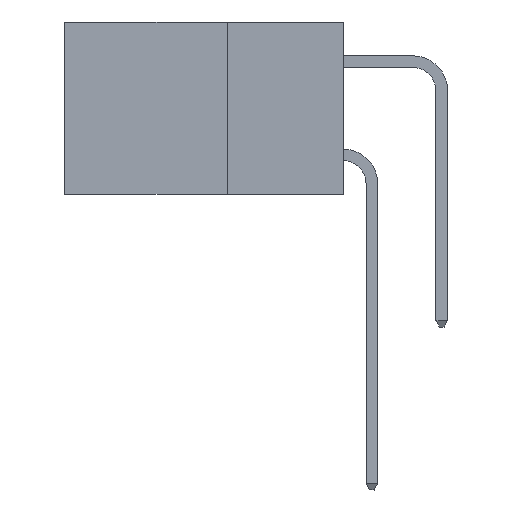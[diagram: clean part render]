
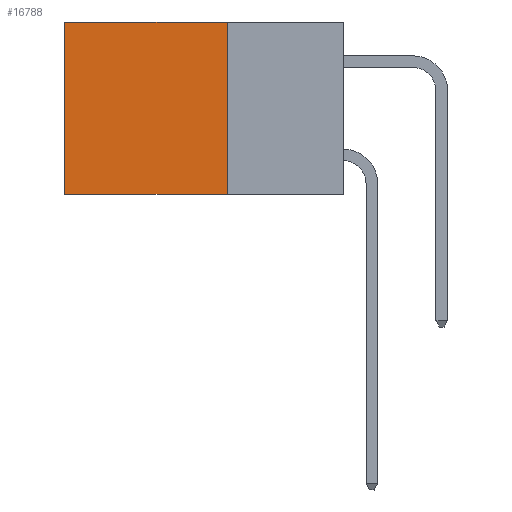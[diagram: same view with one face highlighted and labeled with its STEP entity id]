
A CAD part, left-side view. The second image highlights one B-rep face of the part: STEP entity #16788.
In plain terms, the highlighted planar face has unit normal (-1, 0, 0).
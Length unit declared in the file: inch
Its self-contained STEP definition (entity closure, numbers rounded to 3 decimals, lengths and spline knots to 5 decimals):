
#1310 = LINE ( 'NONE', #8228, #8907 ) ;
#1550 = LINE ( 'NONE', #19549, #5962 ) ;
#3132 = DIRECTION ( 'NONE',  ( 1., 0., 0. ) ) ;
#3649 = LINE ( 'NONE', #10233, #14869 ) ;
#4158 = VERTEX_POINT ( 'NONE', #5997 ) ;
#5188 = EDGE_CURVE ( 'NONE', #4158, #20135, #3649, .T. ) ;
#5937 = ORIENTED_EDGE ( 'NONE', *, *, #24723, .F. ) ;
#5962 = VECTOR ( 'NONE', #19629, 39.37008 ) ;
#5997 = CARTESIAN_POINT ( 'NONE',  ( 0.298, 0.25, 0. ) ) ;
#6469 = CARTESIAN_POINT ( 'NONE',  ( 0.298, 0.6, 0. ) ) ;
#6713 = DIRECTION ( 'NONE',  ( 0., 0., -1. ) ) ;
#6956 = VECTOR ( 'NONE', #21360, 39.37008 ) ;
#8228 = CARTESIAN_POINT ( 'NONE',  ( 0.298, 0.25, -0.37 ) ) ;
#8318 = DIRECTION ( 'NONE',  ( 0., 1., 0. ) ) ;
#8907 = VECTOR ( 'NONE', #8318, 39.37008 ) ;
#10233 = CARTESIAN_POINT ( 'NONE',  ( 0.298, 0.25, 0. ) ) ;
#10533 = VERTEX_POINT ( 'NONE', #6469 ) ;
#11574 = FACE_OUTER_BOUND ( 'NONE', #25048, .T. ) ;
#12467 = CARTESIAN_POINT ( 'NONE',  ( 0.298, 0.25, -0.37 ) ) ;
#12983 = PLANE ( 'NONE',  #14633 ) ;
#13127 = ORIENTED_EDGE ( 'NONE', *, *, #15025, .T. ) ;
#14633 = AXIS2_PLACEMENT_3D ( 'NONE', #20948, #3132, #19202 ) ;
#14869 = VECTOR ( 'NONE', #6713, 39.37008 ) ;
#15025 = EDGE_CURVE ( 'NONE', #4158, #10533, #17299, .T. ) ;
#16788 = ADVANCED_FACE ( 'NONE', ( #11574 ), #12983, .F. ) ;
#16863 = ORIENTED_EDGE ( 'NONE', *, *, #19652, .T. ) ;
#17299 = LINE ( 'NONE', #21227, #6956 ) ;
#19202 = DIRECTION ( 'NONE',  ( 0., 0., -1. ) ) ;
#19549 = CARTESIAN_POINT ( 'NONE',  ( 0.298, 0.6, 0. ) ) ;
#19629 = DIRECTION ( 'NONE',  ( 0., 0., -1. ) ) ;
#19652 = EDGE_CURVE ( 'NONE', #10533, #21621, #1550, .T. ) ;
#19852 = ORIENTED_EDGE ( 'NONE', *, *, #5188, .F. ) ;
#20135 = VERTEX_POINT ( 'NONE', #12467 ) ;
#20948 = CARTESIAN_POINT ( 'NONE',  ( 0.298, 0.25, 0. ) ) ;
#21227 = CARTESIAN_POINT ( 'NONE',  ( 0.298, 0.25, 0. ) ) ;
#21360 = DIRECTION ( 'NONE',  ( 0., 1., 0. ) ) ;
#21621 = VERTEX_POINT ( 'NONE', #24639 ) ;
#24639 = CARTESIAN_POINT ( 'NONE',  ( 0.298, 0.6, -0.37 ) ) ;
#24723 = EDGE_CURVE ( 'NONE', #20135, #21621, #1310, .T. ) ;
#25048 = EDGE_LOOP ( 'NONE', ( #16863, #5937, #19852, #13127 ) ) ;
